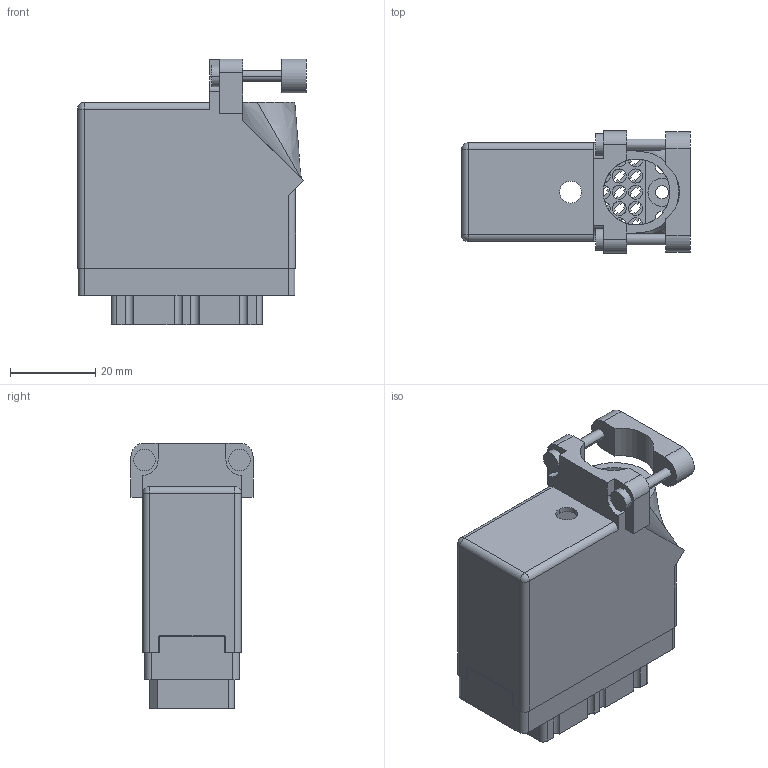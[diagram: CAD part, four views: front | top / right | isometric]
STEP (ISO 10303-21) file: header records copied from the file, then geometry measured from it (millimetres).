
FILE_DESCRIPTION (( 'STEP AP203' ), '1' );
FILE_NAME ('519-036-000-430.STEP', '2020-09-09T19:53:56', ( '' ), ( '' ), 'SwSTEP 2.0', 'SolidWorks 2020', '' );
FILE_SCHEMA (( 'CONFIG_CONTROL_DESIGN' ));
Length unit declared in the file: inch
Products named in the file (3): 519-036-000-430; 516-230-001_Plastic - 038 Top Entry - Large Clamp; 519 Receptacle Insulator_036
Assembly tree (2 placements, depth 2):
  519-036-000-430
    519 Receptacle Insulator_036
    516-230-001_Plastic - 038 Top Entry - Large Clamp
Bounding box: 53.62 x 28.57 x 62.26 mm (x, y, z)
Volume: 22325.7 mm3; surface area: 28414.5 mm2
Topology: 2 solids, 2 shells, 928 faces, 2701 edges, 1796 vertices
Faces by surface type: plane 656, cylinder 265, bspline 3, cone 2, sphere 2
Entity records: 31203 total; most frequent: CARTESIAN_POINT 5521, ORIENTED_EDGE 5398, DIRECTION 5228, EDGE_CURVE 2699, LINE 2022, VECTOR 2022, VERTEX_POINT 1796, AXIS2_PLACEMENT_3D 1603
